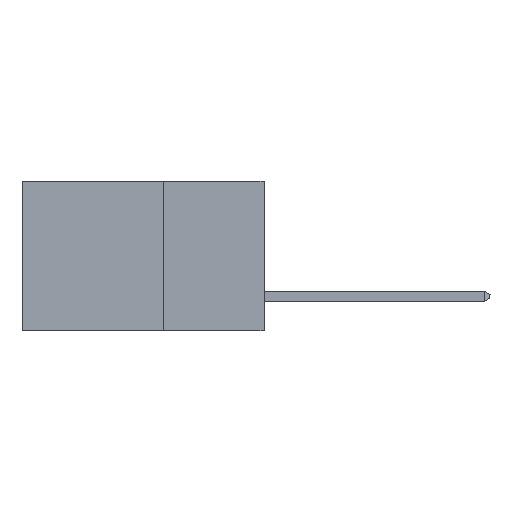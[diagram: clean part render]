
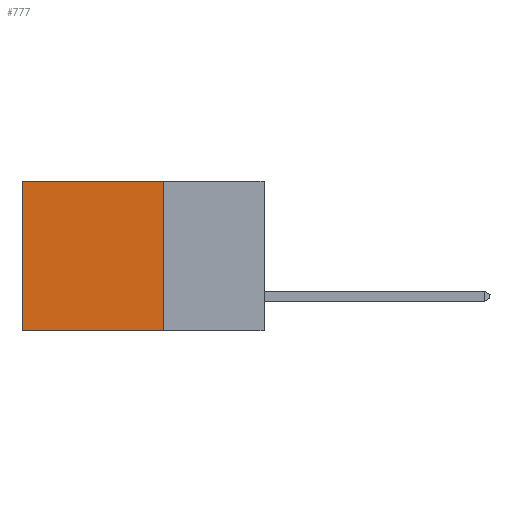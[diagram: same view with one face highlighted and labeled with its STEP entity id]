
A CAD part, left-side view. The second image highlights one B-rep face of the part: STEP entity #777.
In plain terms, the highlighted planar face has unit normal (-1, 0, 0).
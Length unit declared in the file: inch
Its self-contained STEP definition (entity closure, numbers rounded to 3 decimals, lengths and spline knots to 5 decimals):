
#706 = EDGE_LOOP ( 'NONE', ( #7504, #11718, #6613, #4724 ) ) ;
#752 = VERTEX_POINT ( 'NONE', #14968 ) ;
#777 = ADVANCED_FACE ( 'NONE', ( #12344 ), #6586, .F. ) ;
#1436 = DIRECTION ( 'NONE',  ( 0., 0., -1. ) ) ;
#1662 = CARTESIAN_POINT ( 'NONE',  ( 0.298, 0.6, 0. ) ) ;
#2376 = DIRECTION ( 'NONE',  ( 1., 0., 0. ) ) ;
#3160 = VERTEX_POINT ( 'NONE', #14019 ) ;
#3793 = DIRECTION ( 'NONE',  ( 0., 0., -1. ) ) ;
#4724 = ORIENTED_EDGE ( 'NONE', *, *, #17990, .T. ) ;
#5692 = CARTESIAN_POINT ( 'NONE',  ( 0.298, 0.25, 0. ) ) ;
#6586 = PLANE ( 'NONE',  #8980 ) ;
#6613 = ORIENTED_EDGE ( 'NONE', *, *, #16660, .F. ) ;
#7504 = ORIENTED_EDGE ( 'NONE', *, *, #14425, .T. ) ;
#7588 = VERTEX_POINT ( 'NONE', #1662 ) ;
#8409 = VERTEX_POINT ( 'NONE', #17682 ) ;
#8410 = DIRECTION ( 'NONE',  ( 0., 0., -1. ) ) ;
#8697 = VECTOR ( 'NONE', #1436, 39.37008 ) ;
#8980 = AXIS2_PLACEMENT_3D ( 'NONE', #9279, #2376, #3793 ) ;
#9066 = LINE ( 'NONE', #5692, #12413 ) ;
#9279 = CARTESIAN_POINT ( 'NONE',  ( 0.298, 0.25, 0. ) ) ;
#9895 = CARTESIAN_POINT ( 'NONE',  ( 0.298, 0.25, 0. ) ) ;
#11718 = ORIENTED_EDGE ( 'NONE', *, *, #16220, .F. ) ;
#12344 = FACE_OUTER_BOUND ( 'NONE', #706, .T. ) ;
#12413 = VECTOR ( 'NONE', #16036, 39.37008 ) ;
#14019 = CARTESIAN_POINT ( 'NONE',  ( 0.298, 0.25, -0.37 ) ) ;
#14052 = LINE ( 'NONE', #15352, #17791 ) ;
#14337 = VECTOR ( 'NONE', #8410, 39.37008 ) ;
#14425 = EDGE_CURVE ( 'NONE', #7588, #752, #17874, .T. ) ;
#14449 = LINE ( 'NONE', #9895, #8697 ) ;
#14968 = CARTESIAN_POINT ( 'NONE',  ( 0.298, 0.6, -0.37 ) ) ;
#15352 = CARTESIAN_POINT ( 'NONE',  ( 0.298, 0.25, -0.37 ) ) ;
#15458 = CARTESIAN_POINT ( 'NONE',  ( 0.298, 0.6, 0. ) ) ;
#15596 = DIRECTION ( 'NONE',  ( 0., 1., 0. ) ) ;
#16036 = DIRECTION ( 'NONE',  ( 0., 1., 0. ) ) ;
#16220 = EDGE_CURVE ( 'NONE', #3160, #752, #14052, .T. ) ;
#16660 = EDGE_CURVE ( 'NONE', #8409, #3160, #14449, .T. ) ;
#17682 = CARTESIAN_POINT ( 'NONE',  ( 0.298, 0.25, 0. ) ) ;
#17791 = VECTOR ( 'NONE', #15596, 39.37008 ) ;
#17874 = LINE ( 'NONE', #15458, #14337 ) ;
#17990 = EDGE_CURVE ( 'NONE', #8409, #7588, #9066, .T. ) ;
